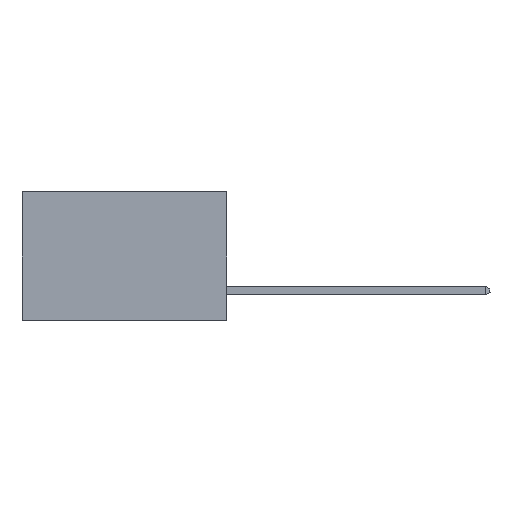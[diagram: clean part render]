
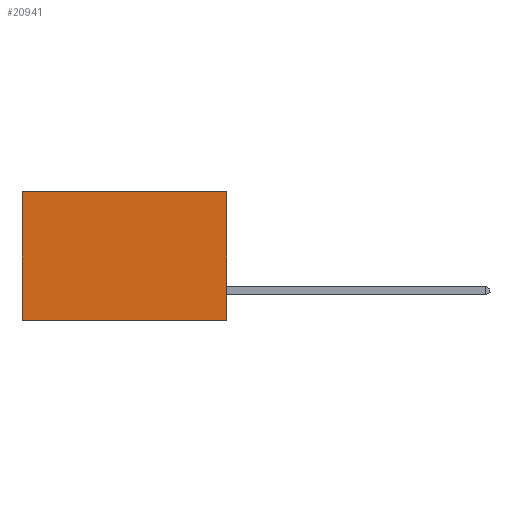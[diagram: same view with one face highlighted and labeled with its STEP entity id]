
A CAD part, left-side view. The second image highlights one B-rep face of the part: STEP entity #20941.
In plain terms, the highlighted planar face has unit normal (-1, 0, 0).
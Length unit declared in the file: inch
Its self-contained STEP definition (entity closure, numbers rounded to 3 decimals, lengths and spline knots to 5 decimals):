
#1 = CARTESIAN_POINT ( 'NONE',  ( 0.277, 0., -0.37 ) ) ;
#555 = LINE ( 'NONE', #15636, #21749 ) ;
#1511 = VECTOR ( 'NONE', #18550, 39.37008 ) ;
#2120 = DIRECTION ( 'NONE',  ( 0., 0., -1. ) ) ;
#2161 = FACE_OUTER_BOUND ( 'NONE', #23714, .T. ) ;
#3300 = CARTESIAN_POINT ( 'NONE',  ( 0.277, 0., 0. ) ) ;
#4522 = VECTOR ( 'NONE', #8335, 39.37008 ) ;
#5521 = EDGE_CURVE ( 'NONE', #21879, #22968, #26231, .T. ) ;
#5861 = AXIS2_PLACEMENT_3D ( 'NONE', #1, #14894, #2120 ) ;
#5914 = VECTOR ( 'NONE', #12200, 39.37008 ) ;
#7853 = LINE ( 'NONE', #7982, #1511 ) ;
#7982 = CARTESIAN_POINT ( 'NONE',  ( 0.277, 0., 0. ) ) ;
#8315 = CARTESIAN_POINT ( 'NONE',  ( 0.277, 0.59, -0.37 ) ) ;
#8335 = DIRECTION ( 'NONE',  ( 0., 0., -1. ) ) ;
#9190 = EDGE_CURVE ( 'NONE', #17480, #22968, #555, .T. ) ;
#9361 = CARTESIAN_POINT ( 'NONE',  ( 0.277, 0.59, -0.37 ) ) ;
#10037 = CARTESIAN_POINT ( 'NONE',  ( 0.277, 0., -0.37 ) ) ;
#10232 = EDGE_CURVE ( 'NONE', #15191, #21879, #7853, .T. ) ;
#10499 = ORIENTED_EDGE ( 'NONE', *, *, #5521, .T. ) ;
#10542 = ORIENTED_EDGE ( 'NONE', *, *, #9190, .F. ) ;
#10632 = PLANE ( 'NONE',  #5861 ) ;
#12200 = DIRECTION ( 'NONE',  ( 0., 0., -1. ) ) ;
#12277 = LINE ( 'NONE', #10037, #5914 ) ;
#14894 = DIRECTION ( 'NONE',  ( 1., 0., 0. ) ) ;
#15191 = VERTEX_POINT ( 'NONE', #3300 ) ;
#15576 = DIRECTION ( 'NONE',  ( 0., 1., 0. ) ) ;
#15636 = CARTESIAN_POINT ( 'NONE',  ( 0.277, 0., -0.37 ) ) ;
#17480 = VERTEX_POINT ( 'NONE', #20363 ) ;
#18550 = DIRECTION ( 'NONE',  ( 0., 1., 0. ) ) ;
#18688 = EDGE_CURVE ( 'NONE', #15191, #17480, #12277, .T. ) ;
#20271 = CARTESIAN_POINT ( 'NONE',  ( 0.277, 0.59, 0. ) ) ;
#20363 = CARTESIAN_POINT ( 'NONE',  ( 0.277, 0., -0.37 ) ) ;
#20570 = ORIENTED_EDGE ( 'NONE', *, *, #10232, .T. ) ;
#20941 = ADVANCED_FACE ( 'NONE', ( #2161 ), #10632, .F. ) ;
#21604 = ORIENTED_EDGE ( 'NONE', *, *, #18688, .F. ) ;
#21749 = VECTOR ( 'NONE', #15576, 39.37008 ) ;
#21879 = VERTEX_POINT ( 'NONE', #20271 ) ;
#22968 = VERTEX_POINT ( 'NONE', #9361 ) ;
#23714 = EDGE_LOOP ( 'NONE', ( #10499, #10542, #21604, #20570 ) ) ;
#26231 = LINE ( 'NONE', #8315, #4522 ) ;
